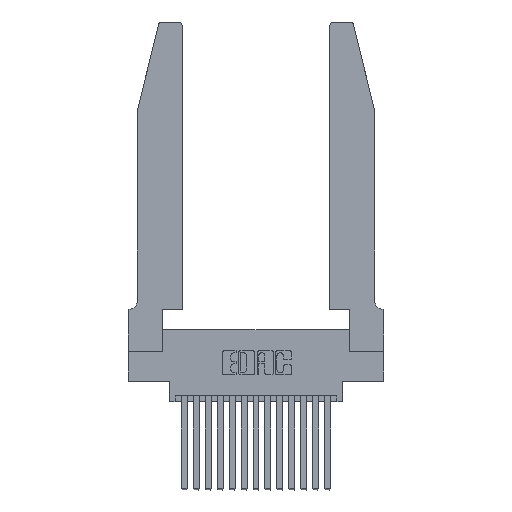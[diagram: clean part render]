
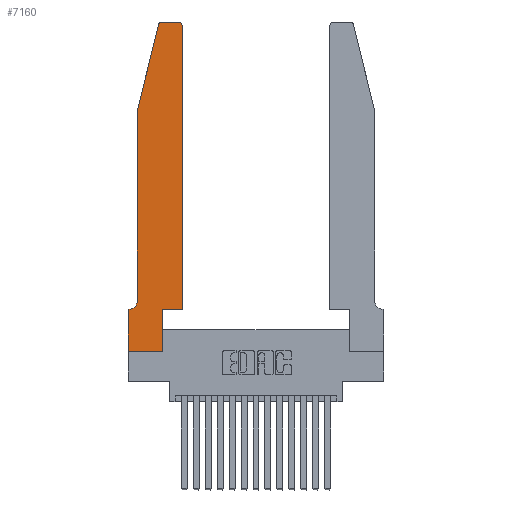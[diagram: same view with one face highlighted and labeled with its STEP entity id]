
A CAD part, top view. The second image highlights one B-rep face of the part: STEP entity #7160.
In plain terms, the highlighted planar face has unit normal (0, 0, 1).
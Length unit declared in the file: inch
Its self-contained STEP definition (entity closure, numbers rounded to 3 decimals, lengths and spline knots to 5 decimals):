
#57 = ORIENTED_EDGE ( 'NONE', *, *, #2376, .T. ) ;
#214 = EDGE_CURVE ( 'NONE', #6098, #3256, #14810, .T. ) ;
#238 = PLANE ( 'NONE',  #12237 ) ;
#499 = VERTEX_POINT ( 'NONE', #10703 ) ;
#546 = ORIENTED_EDGE ( 'NONE', *, *, #13527, .T. ) ;
#1415 = LINE ( 'NONE', #17011, #5363 ) ;
#1752 = DIRECTION ( 'NONE',  ( 1., 0., 0. ) ) ;
#1869 = CARTESIAN_POINT ( 'NONE',  ( 0.2865, 0., 0.37 ) ) ;
#2376 = EDGE_CURVE ( 'NONE', #12685, #499, #18683, .T. ) ;
#2696 = CARTESIAN_POINT ( 'NONE',  ( 0.4505, 2.72, 0.37 ) ) ;
#2846 = DIRECTION ( 'NONE',  ( 0., 0., -1. ) ) ;
#2935 = CARTESIAN_POINT ( 'NONE',  ( 0., 0.35, 0.37 ) ) ;
#2951 = DIRECTION ( 'NONE',  ( 1., 0., 0. ) ) ;
#3009 = FACE_OUTER_BOUND ( 'NONE', #7655, .T. ) ;
#3256 = VERTEX_POINT ( 'NONE', #6088 ) ;
#3324 = EDGE_CURVE ( 'NONE', #14649, #11576, #11584, .T. ) ;
#3583 = DIRECTION ( 'NONE',  ( 0., 1., 0. ) ) ;
#3655 = CIRCLE ( 'NONE', #12376, 0.07 ) ;
#4010 = ORIENTED_EDGE ( 'NONE', *, *, #8817, .T. ) ;
#4527 = VECTOR ( 'NONE', #13672, 39.37008 ) ;
#4741 = VECTOR ( 'NONE', #13544, 39.37008 ) ;
#4915 = VECTOR ( 'NONE', #15008, 39.37008 ) ;
#4998 = LINE ( 'NONE', #10807, #4527 ) ;
#5363 = VECTOR ( 'NONE', #6988, 39.37008 ) ;
#5364 = DIRECTION ( 'NONE',  ( 0., -1., 0. ) ) ;
#5824 = EDGE_CURVE ( 'NONE', #11576, #16824, #10039, .T. ) ;
#5911 = ORIENTED_EDGE ( 'NONE', *, *, #5824, .T. ) ;
#6045 = CARTESIAN_POINT ( 'NONE',  ( 0.284, 2.72, 0.37 ) ) ;
#6088 = CARTESIAN_POINT ( 'NONE',  ( 0., 0., 0.37 ) ) ;
#6098 = VERTEX_POINT ( 'NONE', #2935 ) ;
#6311 = CARTESIAN_POINT ( 'NONE',  ( 0.4505, 0.35, 0.37 ) ) ;
#6606 = EDGE_CURVE ( 'NONE', #7260, #14340, #1415, .T. ) ;
#6797 = AXIS2_PLACEMENT_3D ( 'NONE', #6045, #16113, #7527 ) ;
#6890 = DIRECTION ( 'NONE',  ( 0., 0., 1. ) ) ;
#6988 = DIRECTION ( 'NONE',  ( 0., 1., 0. ) ) ;
#7042 = CARTESIAN_POINT ( 'NONE',  ( 0.0755, 2., 0.37 ) ) ;
#7160 = ADVANCED_FACE ( 'NONE', ( #3009 ), #238, .T. ) ;
#7260 = VERTEX_POINT ( 'NONE', #1869 ) ;
#7290 = VECTOR ( 'NONE', #10585, 39.37008 ) ;
#7527 = DIRECTION ( 'NONE',  ( 1., 0., 0. ) ) ;
#7655 = EDGE_LOOP ( 'NONE', ( #10511, #10973, #14747, #57, #4010, #546, #8475, #12314, #8929, #12760, #16942, #5911 ) ) ;
#7839 = CARTESIAN_POINT ( 'NONE',  ( 0.0755, 0.35, 0.37 ) ) ;
#7863 = CARTESIAN_POINT ( 'NONE',  ( 0.4505, 0.35, 0.37 ) ) ;
#8475 = ORIENTED_EDGE ( 'NONE', *, *, #214, .T. ) ;
#8817 = EDGE_CURVE ( 'NONE', #499, #17315, #3655, .T. ) ;
#8929 = ORIENTED_EDGE ( 'NONE', *, *, #6606, .T. ) ;
#9158 = CARTESIAN_POINT ( 'NONE',  ( 0., 0.35, 0.37 ) ) ;
#9717 = EDGE_CURVE ( 'NONE', #16824, #18616, #4998, .T. ) ;
#10039 = CIRCLE ( 'NONE', #17427, 0.03 ) ;
#10070 = EDGE_CURVE ( 'NONE', #12241, #12685, #11050, .T. ) ;
#10511 = ORIENTED_EDGE ( 'NONE', *, *, #9717, .T. ) ;
#10576 = VECTOR ( 'NONE', #5364, 39.37008 ) ;
#10585 = DIRECTION ( 'NONE',  ( 0., -1., 0. ) ) ;
#10633 = DIRECTION ( 'NONE',  ( 0., 0., 1. ) ) ;
#10703 = CARTESIAN_POINT ( 'NONE',  ( 0.0755, 0.42, 0.37 ) ) ;
#10702 = LINE ( 'NONE', #15982, #17778 ) ;
#10807 = CARTESIAN_POINT ( 'NONE',  ( 0.2605, 2.75, 0.37 ) ) ;
#10973 = ORIENTED_EDGE ( 'NONE', *, *, #11712, .T. ) ;
#11044 = CARTESIAN_POINT ( 'NONE',  ( 0.0755, 2., 0.37 ) ) ;
#11050 = LINE ( 'NONE', #11044, #14383 ) ;
#11576 = VERTEX_POINT ( 'NONE', #2696 ) ;
#11584 = LINE ( 'NONE', #12023, #12028 ) ;
#11698 = CARTESIAN_POINT ( 'NONE',  ( 0.0055, 0.42, 0.37 ) ) ;
#11712 = EDGE_CURVE ( 'NONE', #18616, #12241, #17658, .T. ) ;
#11842 = EDGE_CURVE ( 'NONE', #14340, #14649, #12575, .T. ) ;
#11862 = CARTESIAN_POINT ( 'NONE',  ( 0., 0., 0.37 ) ) ;
#12023 = CARTESIAN_POINT ( 'NONE',  ( 0.4505, 0.35, 0.37 ) ) ;
#12028 = VECTOR ( 'NONE', #3583, 39.37008 ) ;
#12237 = AXIS2_PLACEMENT_3D ( 'NONE', #9158, #10633, #1752 ) ;
#12241 = VERTEX_POINT ( 'NONE', #14696 ) ;
#12276 = CARTESIAN_POINT ( 'NONE',  ( 0.0755, 2., 0.37 ) ) ;
#12314 = ORIENTED_EDGE ( 'NONE', *, *, #15089, .T. ) ;
#12376 = AXIS2_PLACEMENT_3D ( 'NONE', #11698, #2846, #13129 ) ;
#12575 = LINE ( 'NONE', #6311, #4741 ) ;
#12685 = VERTEX_POINT ( 'NONE', #7042 ) ;
#12731 = LINE ( 'NONE', #7839, #4915 ) ;
#12760 = ORIENTED_EDGE ( 'NONE', *, *, #11842, .T. ) ;
#13129 = DIRECTION ( 'NONE',  ( -1., 0., 0. ) ) ;
#13527 = EDGE_CURVE ( 'NONE', #17315, #6098, #12731, .T. ) ;
#13544 = DIRECTION ( 'NONE',  ( 1., 0., 0. ) ) ;
#13672 = DIRECTION ( 'NONE',  ( -1., 0., 0. ) ) ;
#14340 = VERTEX_POINT ( 'NONE', #18599 ) ;
#14383 = VECTOR ( 'NONE', #16726, 39.37008 ) ;
#14538 = CARTESIAN_POINT ( 'NONE',  ( 0.0055, 0.35, 0.37 ) ) ;
#14649 = VERTEX_POINT ( 'NONE', #7863 ) ;
#14696 = CARTESIAN_POINT ( 'NONE',  ( 0.25487, 2.72718, 0.37 ) ) ;
#14747 = ORIENTED_EDGE ( 'NONE', *, *, #10070, .T. ) ;
#14810 = LINE ( 'NONE', #11862, #10576 ) ;
#15008 = DIRECTION ( 'NONE',  ( -1., 0., 0. ) ) ;
#15089 = EDGE_CURVE ( 'NONE', #3256, #7260, #10702, .T. ) ;
#15498 = CARTESIAN_POINT ( 'NONE',  ( 0.4205, 2.72, 0.37 ) ) ;
#15982 = CARTESIAN_POINT ( 'NONE',  ( 0., 0., 0.37 ) ) ;
#16113 = DIRECTION ( 'NONE',  ( 0., 0., 1. ) ) ;
#16207 = CARTESIAN_POINT ( 'NONE',  ( 0.4205, 2.75, 0.37 ) ) ;
#16726 = DIRECTION ( 'NONE',  ( -0.239, -0.971, 0. ) ) ;
#16824 = VERTEX_POINT ( 'NONE', #16207 ) ;
#16910 = DIRECTION ( 'NONE',  ( 1., 0., 0. ) ) ;
#16942 = ORIENTED_EDGE ( 'NONE', *, *, #3324, .T. ) ;
#17011 = CARTESIAN_POINT ( 'NONE',  ( 0.2865, 0.35, 0.37 ) ) ;
#17315 = VERTEX_POINT ( 'NONE', #14538 ) ;
#17427 = AXIS2_PLACEMENT_3D ( 'NONE', #15498, #6890, #16910 ) ;
#17658 = CIRCLE ( 'NONE', #6797, 0.03 ) ;
#17778 = VECTOR ( 'NONE', #2951, 39.37008 ) ;
#18519 = CARTESIAN_POINT ( 'NONE',  ( 0.284, 2.75, 0.37 ) ) ;
#18599 = CARTESIAN_POINT ( 'NONE',  ( 0.2865, 0.35, 0.37 ) ) ;
#18616 = VERTEX_POINT ( 'NONE', #18519 ) ;
#18683 = LINE ( 'NONE', #12276, #7290 ) ;
